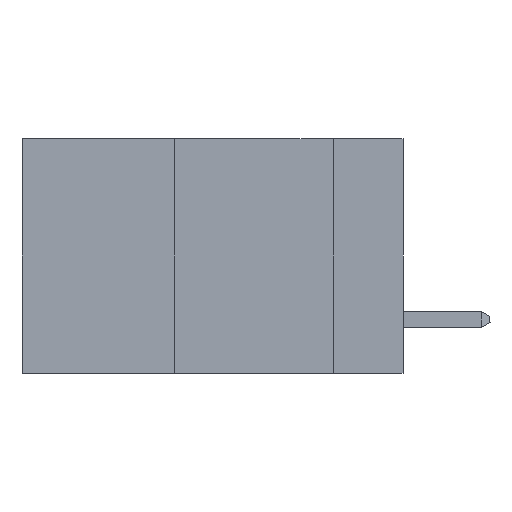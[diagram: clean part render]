
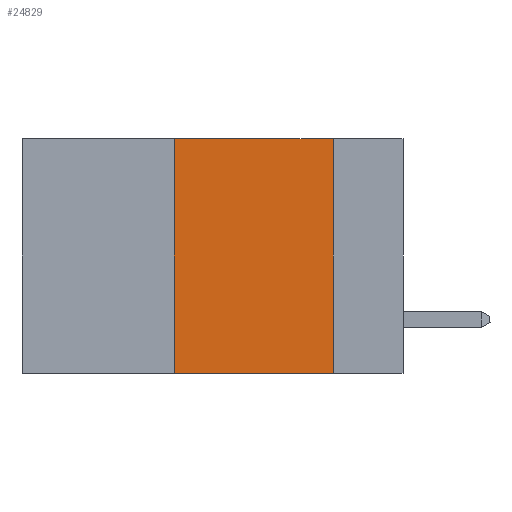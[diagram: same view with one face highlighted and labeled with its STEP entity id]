
A CAD part, left-side view. The second image highlights one B-rep face of the part: STEP entity #24829.
In plain terms, the highlighted planar face has unit normal (-1, 0, 0).
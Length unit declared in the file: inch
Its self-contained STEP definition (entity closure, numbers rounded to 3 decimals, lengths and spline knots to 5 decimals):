
#1148 = DIRECTION ( 'NONE',  ( 0., 0., -1. ) ) ;
#4733 = VECTOR ( 'NONE', #25844, 39.37008 ) ;
#10203 = PLANE ( 'NONE',  #40695 ) ;
#10751 = DIRECTION ( 'NONE',  ( 0., -1., 0. ) ) ;
#11655 = CARTESIAN_POINT ( 'NONE',  ( 0., 0.36, -0.37 ) ) ;
#11677 = CARTESIAN_POINT ( 'NONE',  ( 0., 0.36, 0. ) ) ;
#12850 = LINE ( 'NONE', #44702, #18479 ) ;
#14588 = CARTESIAN_POINT ( 'NONE',  ( 0., 0.11, 0. ) ) ;
#16839 = EDGE_LOOP ( 'NONE', ( #23898, #20833, #43286, #32604 ) ) ;
#16921 = DIRECTION ( 'NONE',  ( 1., 0., 0. ) ) ;
#17568 = CARTESIAN_POINT ( 'NONE',  ( 0., 0.6, 0. ) ) ;
#17858 = EDGE_CURVE ( 'NONE', #46073, #26038, #42664, .T. ) ;
#18479 = VECTOR ( 'NONE', #23167, 39.37008 ) ;
#20833 = ORIENTED_EDGE ( 'NONE', *, *, #28550, .F. ) ;
#23167 = DIRECTION ( 'NONE',  ( 0., -1., 0. ) ) ;
#23838 = FACE_OUTER_BOUND ( 'NONE', #16839, .T. ) ;
#23898 = ORIENTED_EDGE ( 'NONE', *, *, #17858, .F. ) ;
#24715 = VECTOR ( 'NONE', #1148, 39.37008 ) ;
#24829 = ADVANCED_FACE ( 'NONE', ( #23838 ), #10203, .F. ) ;
#25844 = DIRECTION ( 'NONE',  ( 0., 0., 1. ) ) ;
#26038 = VERTEX_POINT ( 'NONE', #33735 ) ;
#28550 = EDGE_CURVE ( 'NONE', #34867, #46073, #46252, .T. ) ;
#29889 = VECTOR ( 'NONE', #10751, 39.37008 ) ;
#29966 = LINE ( 'NONE', #11677, #4733 ) ;
#30171 = EDGE_CURVE ( 'NONE', #39717, #26038, #12850, .T. ) ;
#32604 = ORIENTED_EDGE ( 'NONE', *, *, #30171, .T. ) ;
#33735 = CARTESIAN_POINT ( 'NONE',  ( 0., 0.11, -0.37 ) ) ;
#34802 = CARTESIAN_POINT ( 'NONE',  ( 0., 0.36, 0. ) ) ;
#34867 = VERTEX_POINT ( 'NONE', #34802 ) ;
#36768 = CARTESIAN_POINT ( 'NONE',  ( 0., 0.11, 0. ) ) ;
#39694 = DIRECTION ( 'NONE',  ( 0., 0., -1. ) ) ;
#39717 = VERTEX_POINT ( 'NONE', #11655 ) ;
#40695 = AXIS2_PLACEMENT_3D ( 'NONE', #17568, #16921, #39694 ) ;
#42485 = CARTESIAN_POINT ( 'NONE',  ( 0., 0.6, 0. ) ) ;
#42664 = LINE ( 'NONE', #36768, #24715 ) ;
#43286 = ORIENTED_EDGE ( 'NONE', *, *, #46600, .F. ) ;
#44702 = CARTESIAN_POINT ( 'NONE',  ( 0., 0.6, -0.37 ) ) ;
#46073 = VERTEX_POINT ( 'NONE', #14588 ) ;
#46252 = LINE ( 'NONE', #42485, #29889 ) ;
#46600 = EDGE_CURVE ( 'NONE', #39717, #34867, #29966, .T. ) ;
